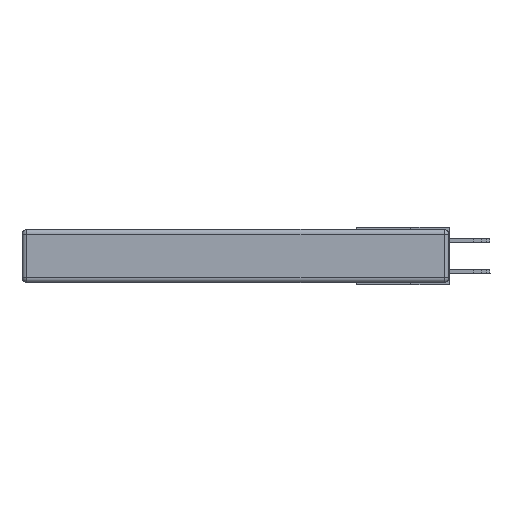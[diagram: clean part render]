
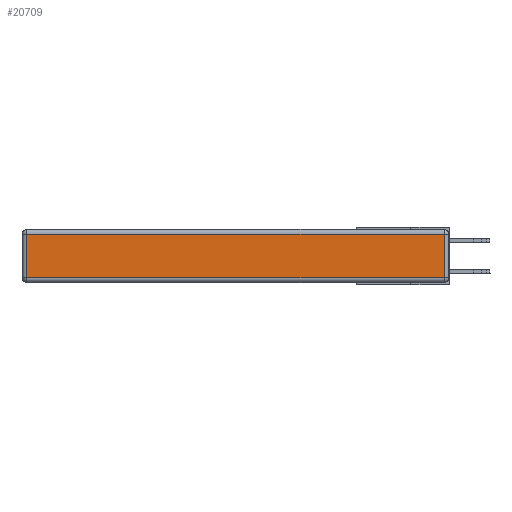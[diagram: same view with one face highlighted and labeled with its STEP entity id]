
A CAD part, left-side view. The second image highlights one B-rep face of the part: STEP entity #20709.
In plain terms, the highlighted planar face has unit normal (-1, 0, 0).
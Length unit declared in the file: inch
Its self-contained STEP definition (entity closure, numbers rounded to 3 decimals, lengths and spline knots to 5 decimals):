
#76 = ORIENTED_EDGE ( 'NONE', *, *, #13756, .T. ) ;
#252 = VECTOR ( 'NONE', #9571, 39.37008 ) ;
#281 = DIRECTION ( 'NONE',  ( 0., 0., -1. ) ) ;
#1086 = FACE_OUTER_BOUND ( 'NONE', #10882, .T. ) ;
#1762 = VERTEX_POINT ( 'NONE', #7894 ) ;
#1920 = CARTESIAN_POINT ( 'NONE',  ( 0., 2.75, -0.03 ) ) ;
#2644 = EDGE_CURVE ( 'NONE', #4681, #1762, #5868, .T. ) ;
#3578 = VECTOR ( 'NONE', #16922, 39.37008 ) ;
#4661 = VERTEX_POINT ( 'NONE', #9644 ) ;
#4681 = VERTEX_POINT ( 'NONE', #7578 ) ;
#5868 = LINE ( 'NONE', #15174, #3578 ) ;
#6863 = LINE ( 'NONE', #1920, #252 ) ;
#7519 = DIRECTION ( 'NONE',  ( 0., 0., 1. ) ) ;
#7578 = CARTESIAN_POINT ( 'NONE',  ( 0., 2.72, -0.313 ) ) ;
#7723 = AXIS2_PLACEMENT_3D ( 'NONE', #13731, #17149, #13810 ) ;
#7894 = CARTESIAN_POINT ( 'NONE',  ( 0., 0.03, -0.313 ) ) ;
#9272 = CARTESIAN_POINT ( 'NONE',  ( 0., 0.03, -0.343 ) ) ;
#9571 = DIRECTION ( 'NONE',  ( 0., 1., 0. ) ) ;
#9644 = CARTESIAN_POINT ( 'NONE',  ( 0., 2.72, -0.03 ) ) ;
#10176 = CARTESIAN_POINT ( 'NONE',  ( 0., 0.03, -0.03 ) ) ;
#10882 = EDGE_LOOP ( 'NONE', ( #15663, #18484, #20378, #76 ) ) ;
#13731 = CARTESIAN_POINT ( 'NONE',  ( 0., 0., -0.343 ) ) ;
#13756 = EDGE_CURVE ( 'NONE', #4661, #4681, #14237, .T. ) ;
#13810 = DIRECTION ( 'NONE',  ( 0., 0., 1. ) ) ;
#14185 = EDGE_CURVE ( 'NONE', #15104, #4661, #6863, .T. ) ;
#14237 = LINE ( 'NONE', #23649, #21123 ) ;
#15104 = VERTEX_POINT ( 'NONE', #10176 ) ;
#15174 = CARTESIAN_POINT ( 'NONE',  ( 0., 0., -0.313 ) ) ;
#15663 = ORIENTED_EDGE ( 'NONE', *, *, #2644, .T. ) ;
#16922 = DIRECTION ( 'NONE',  ( 0., -1., 0. ) ) ;
#17149 = DIRECTION ( 'NONE',  ( -1., 0., 0. ) ) ;
#17366 = VECTOR ( 'NONE', #7519, 39.37008 ) ;
#18484 = ORIENTED_EDGE ( 'NONE', *, *, #19411, .T. ) ;
#19076 = PLANE ( 'NONE',  #7723 ) ;
#19411 = EDGE_CURVE ( 'NONE', #1762, #15104, #22230, .T. ) ;
#20378 = ORIENTED_EDGE ( 'NONE', *, *, #14185, .T. ) ;
#20709 = ADVANCED_FACE ( 'NONE', ( #1086 ), #19076, .T. ) ;
#21123 = VECTOR ( 'NONE', #281, 39.37008 ) ;
#22230 = LINE ( 'NONE', #9272, #17366 ) ;
#23649 = CARTESIAN_POINT ( 'NONE',  ( 0., 2.72, -0.343 ) ) ;
